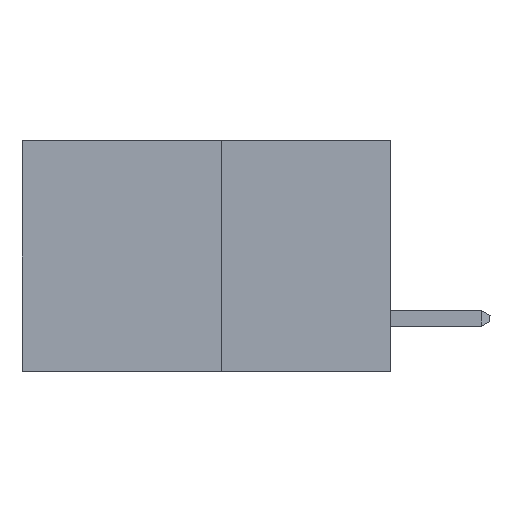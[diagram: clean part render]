
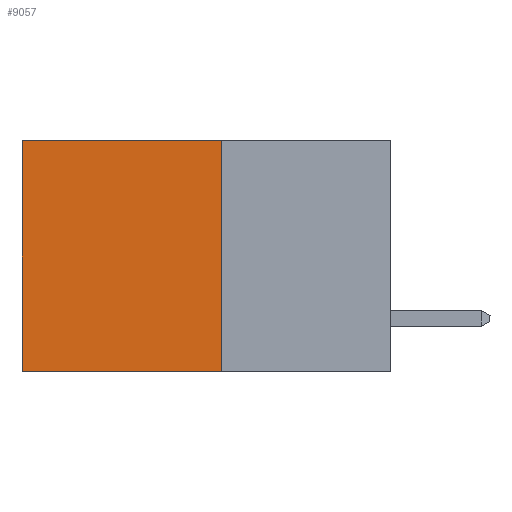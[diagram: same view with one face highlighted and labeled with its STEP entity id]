
A CAD part, left-side view. The second image highlights one B-rep face of the part: STEP entity #9057.
In plain terms, the highlighted planar face has unit normal (-1, 0, 0).
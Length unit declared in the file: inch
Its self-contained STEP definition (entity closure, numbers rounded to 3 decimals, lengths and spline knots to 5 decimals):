
#61 = VECTOR ( 'NONE', #3631, 39.37008 ) ;
#350 = CARTESIAN_POINT ( 'NONE',  ( 0.277, 0.27, -0.37 ) ) ;
#753 = VERTEX_POINT ( 'NONE', #1596 ) ;
#800 = DIRECTION ( 'NONE',  ( 0., 0., -1. ) ) ;
#909 = ORIENTED_EDGE ( 'NONE', *, *, #8192, .T. ) ;
#1138 = DIRECTION ( 'NONE',  ( 0., 0., -1. ) ) ;
#1335 = CARTESIAN_POINT ( 'NONE',  ( 0.277, 0.27, -0.37 ) ) ;
#1596 = CARTESIAN_POINT ( 'NONE',  ( 0.277, 0.59, 0. ) ) ;
#1768 = VERTEX_POINT ( 'NONE', #3685 ) ;
#1886 = LINE ( 'NONE', #9805, #10007 ) ;
#2704 = CARTESIAN_POINT ( 'NONE',  ( 0.277, 0.59, -0.37 ) ) ;
#3262 = ORIENTED_EDGE ( 'NONE', *, *, #6292, .F. ) ;
#3269 = VERTEX_POINT ( 'NONE', #2704 ) ;
#3487 = EDGE_LOOP ( 'NONE', ( #9136, #3635, #3262, #909 ) ) ;
#3631 = DIRECTION ( 'NONE',  ( 0., 0., -1. ) ) ;
#3635 = ORIENTED_EDGE ( 'NONE', *, *, #10017, .F. ) ;
#3644 = LINE ( 'NONE', #8498, #7876 ) ;
#3685 = CARTESIAN_POINT ( 'NONE',  ( 0.277, 0.27, 0. ) ) ;
#4066 = VERTEX_POINT ( 'NONE', #1335 ) ;
#4519 = DIRECTION ( 'NONE',  ( 0., 1., 0. ) ) ;
#4702 = CARTESIAN_POINT ( 'NONE',  ( 0.277, 0.27, -0.37 ) ) ;
#5108 = LINE ( 'NONE', #350, #9064 ) ;
#5516 = DIRECTION ( 'NONE',  ( 1., 0., 0. ) ) ;
#5814 = FACE_OUTER_BOUND ( 'NONE', #3487, .T. ) ;
#5837 = AXIS2_PLACEMENT_3D ( 'NONE', #4702, #5516, #800 ) ;
#6292 = EDGE_CURVE ( 'NONE', #1768, #4066, #5108, .T. ) ;
#7527 = DIRECTION ( 'NONE',  ( 0., 1., 0. ) ) ;
#7700 = EDGE_CURVE ( 'NONE', #753, #3269, #8224, .T. ) ;
#7876 = VECTOR ( 'NONE', #4519, 39.37008 ) ;
#8192 = EDGE_CURVE ( 'NONE', #1768, #753, #1886, .T. ) ;
#8224 = LINE ( 'NONE', #9921, #61 ) ;
#8498 = CARTESIAN_POINT ( 'NONE',  ( 0.277, 0.27, -0.37 ) ) ;
#9057 = ADVANCED_FACE ( 'NONE', ( #5814 ), #10188, .F. ) ;
#9064 = VECTOR ( 'NONE', #1138, 39.37008 ) ;
#9136 = ORIENTED_EDGE ( 'NONE', *, *, #7700, .T. ) ;
#9805 = CARTESIAN_POINT ( 'NONE',  ( 0.277, 0.27, 0. ) ) ;
#9921 = CARTESIAN_POINT ( 'NONE',  ( 0.277, 0.59, -0.37 ) ) ;
#10007 = VECTOR ( 'NONE', #7527, 39.37008 ) ;
#10017 = EDGE_CURVE ( 'NONE', #4066, #3269, #3644, .T. ) ;
#10188 = PLANE ( 'NONE',  #5837 ) ;
